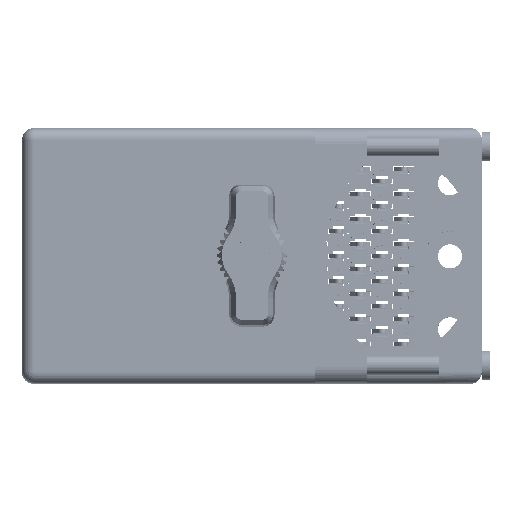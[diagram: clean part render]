
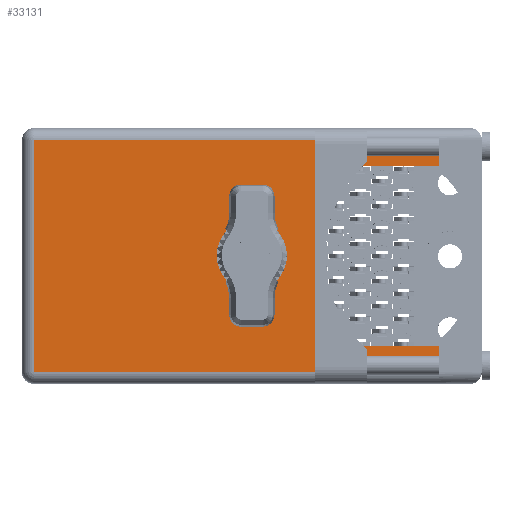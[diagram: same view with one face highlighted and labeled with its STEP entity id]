
A CAD part, top view. The second image highlights one B-rep face of the part: STEP entity #33131.
In plain terms, the highlighted face is planar.
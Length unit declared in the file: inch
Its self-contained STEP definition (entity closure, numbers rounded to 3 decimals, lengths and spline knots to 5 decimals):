
#732 = CARTESIAN_POINT ( 'NONE',  ( -1.3075, 1.93, -0.695 ) ) ;
#2452 = VECTOR ( 'NONE', #46110, 39.37008 ) ;
#3236 = ORIENTED_EDGE ( 'NONE', *, *, #93822, .T. ) ;
#3835 = VERTEX_POINT ( 'NONE', #60736 ) ;
#5745 = VERTEX_POINT ( 'NONE', #11819 ) ;
#7356 = CARTESIAN_POINT ( 'NONE',  ( -1.3775, 1.93, -0.765 ) ) ;
#7708 = DIRECTION ( 'NONE',  ( 0., 1., 0. ) ) ;
#9387 = EDGE_CURVE ( 'NONE', #90686, #67743, #34198, .T. ) ;
#10775 = DIRECTION ( 'NONE',  ( 0., 0., 1. ) ) ;
#11165 = CARTESIAN_POINT ( 'NONE',  ( 1.1215, 1.93, 0.695 ) ) ;
#11819 = CARTESIAN_POINT ( 'NONE',  ( 1.1215, 1.93, -0.54 ) ) ;
#13965 = EDGE_CURVE ( 'NONE', #67743, #5745, #45569, .T. ) ;
#16076 = VECTOR ( 'NONE', #77200, 39.37008 ) ;
#17486 = CIRCLE ( 'NONE', #57946, 0.17 ) ;
#18377 = EDGE_CURVE ( 'NONE', #37196, #3835, #34575, .T. ) ;
#20676 = VECTOR ( 'NONE', #32837, 39.37008 ) ;
#20894 = AXIS2_PLACEMENT_3D ( 'NONE', #7356, #7708, #65065 ) ;
#21979 = ORIENTED_EDGE ( 'NONE', *, *, #91191, .F. ) ;
#22059 = CARTESIAN_POINT ( 'NONE',  ( 1.1215, 1.93, 0.695 ) ) ;
#22077 = CARTESIAN_POINT ( 'NONE',  ( 1.1215, 1.93, -0.54 ) ) ;
#22290 = CARTESIAN_POINT ( 'NONE',  ( 0.4075, 1.93, -0.54 ) ) ;
#22637 = DIRECTION ( 'NONE',  ( 0., 0., -1. ) ) ;
#23018 = CARTESIAN_POINT ( 'NONE',  ( -1.3075, 1.93, -0.765 ) ) ;
#24813 = LINE ( 'NONE', #83748, #46528 ) ;
#25875 = VERTEX_POINT ( 'NONE', #22059 ) ;
#26563 = CARTESIAN_POINT ( 'NONE',  ( 0., 1.93, -0.17 ) ) ;
#27139 = CARTESIAN_POINT ( 'NONE',  ( 1.1215, 1.93, -0.765 ) ) ;
#29445 = VERTEX_POINT ( 'NONE', #38334 ) ;
#32837 = DIRECTION ( 'NONE',  ( 1., 0., 0. ) ) ;
#33131 = ADVANCED_FACE ( 'NONE', ( #98926, #54434 ), #48425, .T. ) ;
#33300 = ORIENTED_EDGE ( 'NONE', *, *, #9387, .T. ) ;
#33672 = CARTESIAN_POINT ( 'NONE',  ( 1.1215, 1.93, -0.765 ) ) ;
#34198 = LINE ( 'NONE', #22290, #53260 ) ;
#34575 = LINE ( 'NONE', #23018, #70123 ) ;
#35083 = ORIENTED_EDGE ( 'NONE', *, *, #47830, .F. ) ;
#37086 = LINE ( 'NONE', #76046, #2452 ) ;
#37196 = VERTEX_POINT ( 'NONE', #732 ) ;
#38054 = DIRECTION ( 'NONE',  ( 0., 0., 1. ) ) ;
#38334 = CARTESIAN_POINT ( 'NONE',  ( 1.1215, 1.93, 0.54 ) ) ;
#38471 = VERTEX_POINT ( 'NONE', #41462 ) ;
#41303 = AXIS2_PLACEMENT_3D ( 'NONE', #56640, #89062, #96567 ) ;
#41462 = CARTESIAN_POINT ( 'NONE',  ( 0., 1.93, 0.17 ) ) ;
#41672 = DIRECTION ( 'NONE',  ( -1., 0., 0. ) ) ;
#42539 = ORIENTED_EDGE ( 'NONE', *, *, #53667, .T. ) ;
#43253 = CARTESIAN_POINT ( 'NONE',  ( 0., 1.93, 0. ) ) ;
#45569 = LINE ( 'NONE', #22077, #20676 ) ;
#45704 = EDGE_CURVE ( 'NONE', #51047, #38471, #17486, .T. ) ;
#46110 = DIRECTION ( 'NONE',  ( -1., 0., 0. ) ) ;
#46122 = ORIENTED_EDGE ( 'NONE', *, *, #73096, .T. ) ;
#46528 = VECTOR ( 'NONE', #41672, 39.37008 ) ;
#47293 = VERTEX_POINT ( 'NONE', #103942 ) ;
#47830 = EDGE_CURVE ( 'NONE', #47293, #5745, #51527, .T. ) ;
#48425 = PLANE ( 'NONE',  #20894 ) ;
#49029 = EDGE_CURVE ( 'NONE', #29445, #25875, #63463, .T. ) ;
#49613 = DIRECTION ( 'NONE',  ( 0., 0., 1. ) ) ;
#51047 = VERTEX_POINT ( 'NONE', #26563 ) ;
#51527 = LINE ( 'NONE', #33672, #80893 ) ;
#53260 = VECTOR ( 'NONE', #22637, 39.37008 ) ;
#53356 = VECTOR ( 'NONE', #84185, 39.37008 ) ;
#53667 = EDGE_CURVE ( 'NONE', #3835, #25875, #59396, .T. ) ;
#54434 = FACE_BOUND ( 'NONE', #87735, .T. ) ;
#56640 = CARTESIAN_POINT ( 'NONE',  ( 0., 1.93, 0. ) ) ;
#57449 = CARTESIAN_POINT ( 'NONE',  ( 0.4075, 1.93, 0.54 ) ) ;
#57946 = AXIS2_PLACEMENT_3D ( 'NONE', #43253, #59632, #10775 ) ;
#59047 = ORIENTED_EDGE ( 'NONE', *, *, #13965, .T. ) ;
#59396 = LINE ( 'NONE', #11165, #16076 ) ;
#59632 = DIRECTION ( 'NONE',  ( 0., 1., 0. ) ) ;
#60736 = CARTESIAN_POINT ( 'NONE',  ( -1.3075, 1.93, 0.695 ) ) ;
#63463 = LINE ( 'NONE', #27139, #53356 ) ;
#65065 = DIRECTION ( 'NONE',  ( -1., 0., 0. ) ) ;
#67743 = VERTEX_POINT ( 'NONE', #84036 ) ;
#70123 = VECTOR ( 'NONE', #38054, 39.37008 ) ;
#73096 = EDGE_CURVE ( 'NONE', #29445, #90686, #24813, .T. ) ;
#76046 = CARTESIAN_POINT ( 'NONE',  ( -1.3775, 1.93, -0.695 ) ) ;
#76178 = ORIENTED_EDGE ( 'NONE', *, *, #18377, .T. ) ;
#77200 = DIRECTION ( 'NONE',  ( 1., 0., 0. ) ) ;
#78494 = ORIENTED_EDGE ( 'NONE', *, *, #49029, .F. ) ;
#80893 = VECTOR ( 'NONE', #49613, 39.37008 ) ;
#82911 = EDGE_LOOP ( 'NONE', ( #76178, #42539, #78494, #46122, #33300, #59047, #35083, #3236 ) ) ;
#83748 = CARTESIAN_POINT ( 'NONE',  ( 1.1215, 1.93, 0.54 ) ) ;
#84036 = CARTESIAN_POINT ( 'NONE',  ( 0.4075, 1.93, -0.54 ) ) ;
#84185 = DIRECTION ( 'NONE',  ( 0., 0., 1. ) ) ;
#87735 = EDGE_LOOP ( 'NONE', ( #21979, #98488 ) ) ;
#89062 = DIRECTION ( 'NONE',  ( 0., 1., 0. ) ) ;
#90686 = VERTEX_POINT ( 'NONE', #57449 ) ;
#91191 = EDGE_CURVE ( 'NONE', #38471, #51047, #93811, .T. ) ;
#93811 = CIRCLE ( 'NONE', #41303, 0.17 ) ;
#93822 = EDGE_CURVE ( 'NONE', #47293, #37196, #37086, .T. ) ;
#96567 = DIRECTION ( 'NONE',  ( 0., 0., 1. ) ) ;
#98488 = ORIENTED_EDGE ( 'NONE', *, *, #45704, .F. ) ;
#98926 = FACE_OUTER_BOUND ( 'NONE', #82911, .T. ) ;
#103942 = CARTESIAN_POINT ( 'NONE',  ( 1.1215, 1.93, -0.695 ) ) ;
